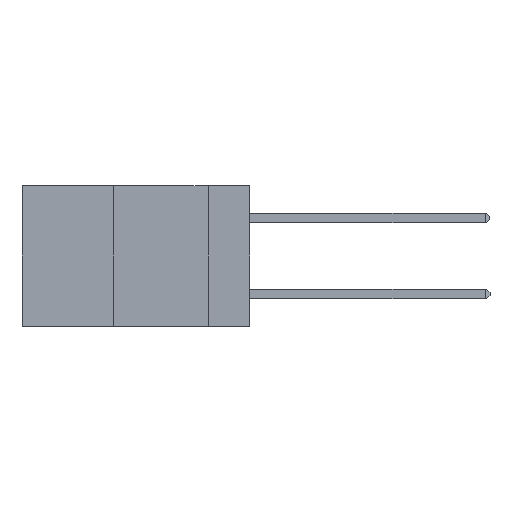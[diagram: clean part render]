
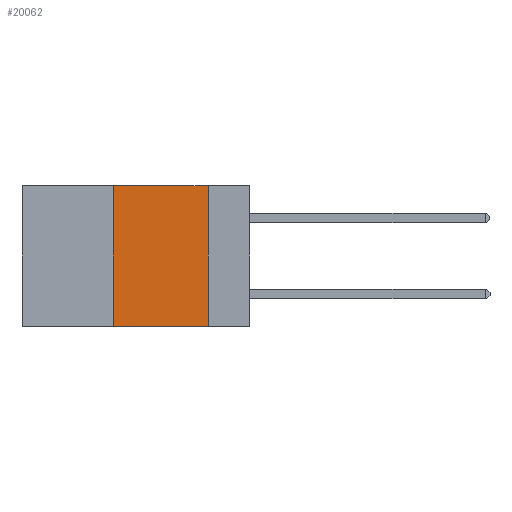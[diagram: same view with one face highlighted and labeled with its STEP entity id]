
A CAD part, left-side view. The second image highlights one B-rep face of the part: STEP entity #20062.
In plain terms, the highlighted planar face has unit normal (-1, 0, 0).
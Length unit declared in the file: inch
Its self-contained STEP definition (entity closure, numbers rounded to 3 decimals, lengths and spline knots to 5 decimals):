
#730 = VERTEX_POINT ( 'NONE', #18269 ) ;
#1084 = CARTESIAN_POINT ( 'NONE',  ( 0., 0.11, 0. ) ) ;
#2657 = DIRECTION ( 'NONE',  ( 0., -1., 0. ) ) ;
#2678 = VECTOR ( 'NONE', #22153, 39.37008 ) ;
#2977 = LINE ( 'NONE', #8908, #2678 ) ;
#3401 = EDGE_CURVE ( 'NONE', #17657, #16163, #16748, .T. ) ;
#3969 = VECTOR ( 'NONE', #21804, 39.37008 ) ;
#4248 = DIRECTION ( 'NONE',  ( 0., 0., -1. ) ) ;
#6064 = PLANE ( 'NONE',  #13319 ) ;
#8043 = VECTOR ( 'NONE', #2657, 39.37008 ) ;
#8797 = CARTESIAN_POINT ( 'NONE',  ( 0., 0.6, 0. ) ) ;
#8908 = CARTESIAN_POINT ( 'NONE',  ( 0., 0.36, 0. ) ) ;
#10733 = DIRECTION ( 'NONE',  ( 0., -1., 0. ) ) ;
#11695 = VECTOR ( 'NONE', #10733, 39.37008 ) ;
#11915 = LINE ( 'NONE', #15896, #8043 ) ;
#13319 = AXIS2_PLACEMENT_3D ( 'NONE', #17596, #21472, #4248 ) ;
#13512 = EDGE_CURVE ( 'NONE', #23459, #17657, #2977, .T. ) ;
#14909 = LINE ( 'NONE', #1084, #3969 ) ;
#15833 = EDGE_CURVE ( 'NONE', #16163, #730, #14909, .T. ) ;
#15896 = CARTESIAN_POINT ( 'NONE',  ( 0., 0.6, -0.37 ) ) ;
#15918 = CARTESIAN_POINT ( 'NONE',  ( 0., 0.36, -0.37 ) ) ;
#16163 = VERTEX_POINT ( 'NONE', #19155 ) ;
#16180 = ORIENTED_EDGE ( 'NONE', *, *, #16759, .T. ) ;
#16748 = LINE ( 'NONE', #8797, #11695 ) ;
#16759 = EDGE_CURVE ( 'NONE', #23459, #730, #11915, .T. ) ;
#17374 = CARTESIAN_POINT ( 'NONE',  ( 0., 0.36, 0. ) ) ;
#17596 = CARTESIAN_POINT ( 'NONE',  ( 0., 0.6, 0. ) ) ;
#17657 = VERTEX_POINT ( 'NONE', #17374 ) ;
#18269 = CARTESIAN_POINT ( 'NONE',  ( 0., 0.11, -0.37 ) ) ;
#19155 = CARTESIAN_POINT ( 'NONE',  ( 0., 0.11, 0. ) ) ;
#19320 = ORIENTED_EDGE ( 'NONE', *, *, #13512, .F. ) ;
#20062 = ADVANCED_FACE ( 'NONE', ( #22585 ), #6064, .F. ) ;
#21472 = DIRECTION ( 'NONE',  ( 1., 0., 0. ) ) ;
#21804 = DIRECTION ( 'NONE',  ( 0., 0., -1. ) ) ;
#22153 = DIRECTION ( 'NONE',  ( 0., 0., 1. ) ) ;
#22585 = FACE_OUTER_BOUND ( 'NONE', #24059, .T. ) ;
#23459 = VERTEX_POINT ( 'NONE', #15918 ) ;
#23497 = ORIENTED_EDGE ( 'NONE', *, *, #3401, .F. ) ;
#23570 = ORIENTED_EDGE ( 'NONE', *, *, #15833, .F. ) ;
#24059 = EDGE_LOOP ( 'NONE', ( #23570, #23497, #19320, #16180 ) ) ;
